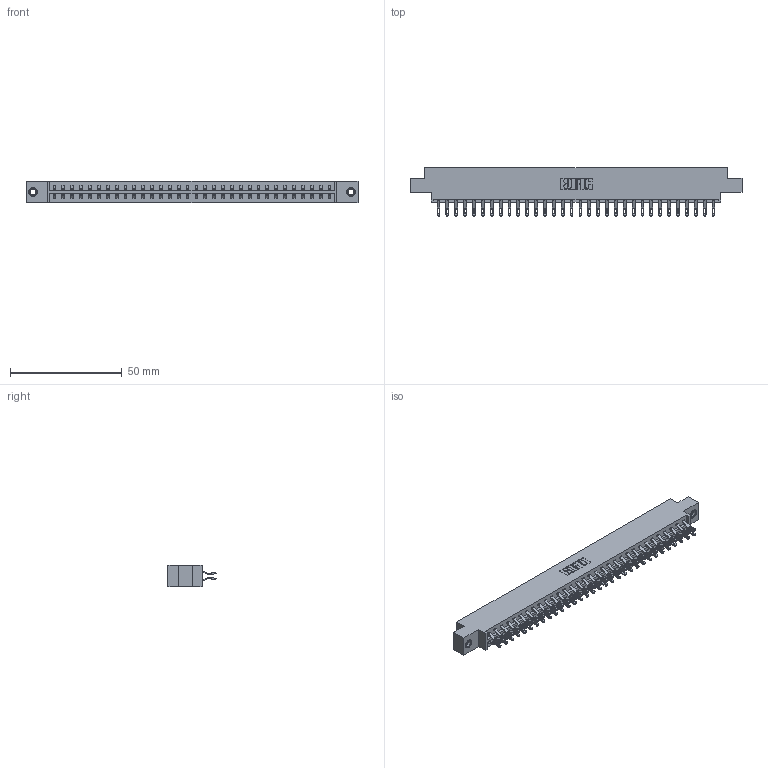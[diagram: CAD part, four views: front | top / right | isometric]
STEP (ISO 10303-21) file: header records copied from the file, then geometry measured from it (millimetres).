
FILE_DESCRIPTION (( 'STEP AP203' ), '1' );
FILE_NAME ('333-064-555-807.STEP', '2018-08-04T10:19:43', ( '' ), ( '' ), 'SwSTEP 2.0', 'SolidWorks 2016', '' );
FILE_SCHEMA (( 'CONFIG_CONTROL_DESIGN' ));
Length unit declared in the file: inch
Products named in the file (4): 333 Part_Offset - .156 Dia - TI; 345-292-001_555 Tail; 345-250-001_345-250-005-103; 333-064-555-807
Assembly tree (67 placements, depth 2):
  333-064-555-807
    333 Part_Offset - .156 Dia - TI
    345-292-001_555 Tail  x64
    345-250-001_345-250-005-103  x2
Bounding box: 148.34 x 21.47 x 9.4 mm (x, y, z)
Volume: 14995.1 mm3; surface area: 18569.6 mm2
Topology: 67 solids, 67 shells, 3890 faces, 12171 edges, 8106 vertices
Faces by surface type: plane 2282, cylinder 1592, cone 12, torus 4
Entity records: 23524 total; most frequent: CARTESIAN_POINT 3931, ORIENTED_EDGE 3830, DIRECTION 3377, EDGE_CURVE 1915, LINE 1747, VECTOR 1747, VERTEX_POINT 1272, AXIS2_PLACEMENT_3D 815
